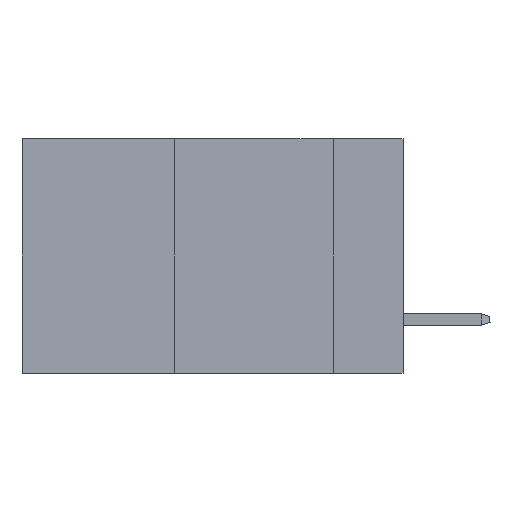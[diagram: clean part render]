
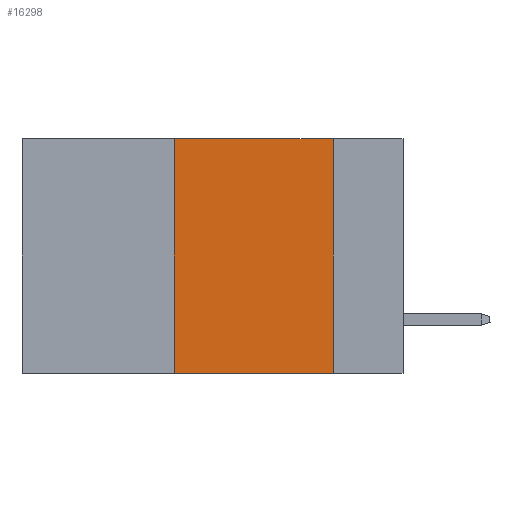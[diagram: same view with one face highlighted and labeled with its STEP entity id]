
A CAD part, left-side view. The second image highlights one B-rep face of the part: STEP entity #16298.
In plain terms, the highlighted planar face has unit normal (-1, 0, 0).
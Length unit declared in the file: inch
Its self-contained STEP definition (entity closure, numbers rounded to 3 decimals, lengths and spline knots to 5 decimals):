
#403 = VERTEX_POINT ( 'NONE', #11159 ) ;
#942 = LINE ( 'NONE', #14309, #24667 ) ;
#1212 = VECTOR ( 'NONE', #13261, 39.37008 ) ;
#4066 = DIRECTION ( 'NONE',  ( 0., 0., 1. ) ) ;
#4519 = ORIENTED_EDGE ( 'NONE', *, *, #20200, .F. ) ;
#5253 = FACE_OUTER_BOUND ( 'NONE', #8256, .T. ) ;
#5329 = ORIENTED_EDGE ( 'NONE', *, *, #18681, .F. ) ;
#6784 = CARTESIAN_POINT ( 'NONE',  ( 0., 0.11, 0. ) ) ;
#8194 = LINE ( 'NONE', #21027, #1212 ) ;
#8256 = EDGE_LOOP ( 'NONE', ( #4519, #19177, #5329, #9972 ) ) ;
#9972 = ORIENTED_EDGE ( 'NONE', *, *, #11150, .T. ) ;
#10637 = CARTESIAN_POINT ( 'NONE',  ( 0., 0.6, 0. ) ) ;
#11150 = EDGE_CURVE ( 'NONE', #403, #21401, #8194, .T. ) ;
#11159 = CARTESIAN_POINT ( 'NONE',  ( 0., 0.36, -0.37 ) ) ;
#13261 = DIRECTION ( 'NONE',  ( 0., -1., 0. ) ) ;
#13306 = PLANE ( 'NONE',  #14883 ) ;
#14121 = DIRECTION ( 'NONE',  ( 0., -1., 0. ) ) ;
#14309 = CARTESIAN_POINT ( 'NONE',  ( 0., 0.6, 0. ) ) ;
#14883 = AXIS2_PLACEMENT_3D ( 'NONE', #10637, #27445, #21937 ) ;
#16143 = CARTESIAN_POINT ( 'NONE',  ( 0., 0.11, 0. ) ) ;
#16298 = ADVANCED_FACE ( 'NONE', ( #5253 ), #13306, .F. ) ;
#17444 = LINE ( 'NONE', #28221, #27979 ) ;
#17792 = VERTEX_POINT ( 'NONE', #6784 ) ;
#18681 = EDGE_CURVE ( 'NONE', #403, #32613, #17444, .T. ) ;
#19177 = ORIENTED_EDGE ( 'NONE', *, *, #21938, .F. ) ;
#20200 = EDGE_CURVE ( 'NONE', #17792, #21401, #27288, .T. ) ;
#21027 = CARTESIAN_POINT ( 'NONE',  ( 0., 0.6, -0.37 ) ) ;
#21401 = VERTEX_POINT ( 'NONE', #27297 ) ;
#21920 = CARTESIAN_POINT ( 'NONE',  ( 0., 0.36, 0. ) ) ;
#21937 = DIRECTION ( 'NONE',  ( 0., 0., -1. ) ) ;
#21938 = EDGE_CURVE ( 'NONE', #32613, #17792, #942, .T. ) ;
#24667 = VECTOR ( 'NONE', #14121, 39.37008 ) ;
#27288 = LINE ( 'NONE', #16143, #33168 ) ;
#27297 = CARTESIAN_POINT ( 'NONE',  ( 0., 0.11, -0.37 ) ) ;
#27445 = DIRECTION ( 'NONE',  ( 1., 0., 0. ) ) ;
#27979 = VECTOR ( 'NONE', #4066, 39.37008 ) ;
#28221 = CARTESIAN_POINT ( 'NONE',  ( 0., 0.36, 0. ) ) ;
#32613 = VERTEX_POINT ( 'NONE', #21920 ) ;
#32761 = DIRECTION ( 'NONE',  ( 0., 0., -1. ) ) ;
#33168 = VECTOR ( 'NONE', #32761, 39.37008 ) ;
